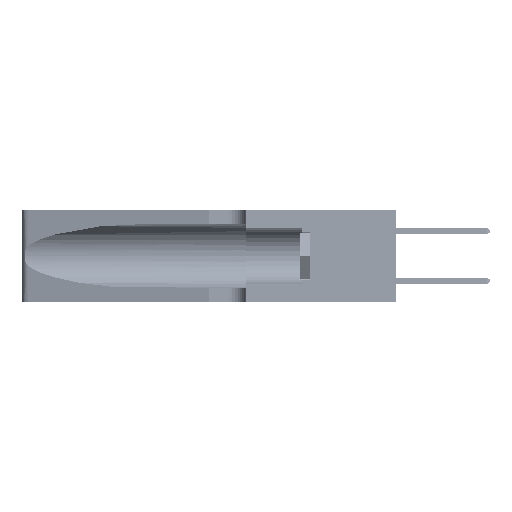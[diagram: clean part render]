
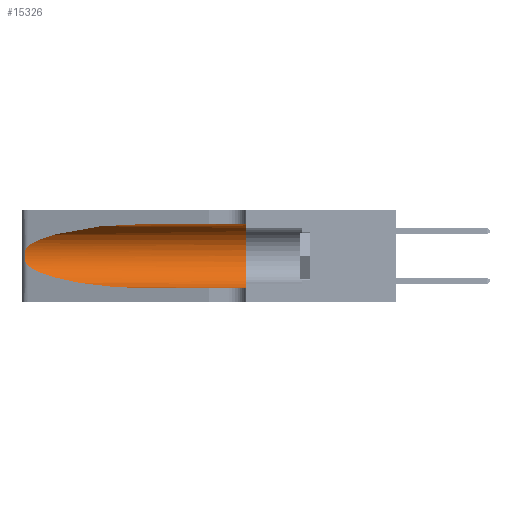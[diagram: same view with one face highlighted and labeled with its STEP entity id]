
A CAD part, left-side view. The second image highlights one B-rep face of the part: STEP entity #15326.
In plain terms, the highlighted cylindrical face has radius 3.308 mm (diameter 6.617 mm), a partial arc.
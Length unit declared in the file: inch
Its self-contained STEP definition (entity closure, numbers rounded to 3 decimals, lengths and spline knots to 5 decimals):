
#369 = CARTESIAN_POINT ( 'NONE',  ( 0.18966, 0.96281, 0.05475 ) ) ;
#538 = AXIS2_PLACEMENT_3D ( 'NONE', #7253, #50254, #26796 ) ;
#1920 = CARTESIAN_POINT ( 'NONE',  ( 0.1305, 0.72297, 0.05475 ) ) ;
#3194 = ORIENTED_EDGE ( 'NONE', *, *, #28924, .T. ) ;
#3664 = ORIENTED_EDGE ( 'NONE', *, *, #30258, .T. ) ;
#4089 = CARTESIAN_POINT ( 'NONE',  ( 0.26075, 1.23896, 0.19203 ) ) ;
#4141 = CARTESIAN_POINT ( 'NONE',  ( 0.25487, 1.22718, 0.14631 ) ) ;
#4428 = CARTESIAN_POINT ( 'NONE',  ( 0.25487, 1.22718, 0.22369 ) ) ;
#5025 = FACE_OUTER_BOUND ( 'NONE', #24819, .T. ) ;
#7253 = CARTESIAN_POINT ( 'NONE',  ( 0.1305, 0.35, 0.185 ) ) ;
#8029 = CARTESIAN_POINT ( 'NONE',  ( 0.25639, 1.23184, 0.21858 ) ) ;
#8126 = EDGE_CURVE ( 'NONE', #20745, #47649, #30087, .T. ) ;
#8811 = VERTEX_POINT ( 'NONE', #24138 ) ;
#9711 = DIRECTION ( 'NONE',  ( 0., -1., 0. ) ) ;
#10299 =( BOUNDED_CURVE ( )  B_SPLINE_CURVE ( 3, ( #44788, #48866, #36911, #29019 ),
 .UNSPECIFIED., .F., .T. ) 
 B_SPLINE_CURVE_WITH_KNOTS ( ( 4, 4 ),
 ( 1.5708, 2.84003 ),
 .UNSPECIFIED. ) 
 CURVE ( )  GEOMETRIC_REPRESENTATION_ITEM ( )  RATIONAL_B_SPLINE_CURVE ( ( 1., 0.87, 0.87, 1. ) ) 
 REPRESENTATION_ITEM ( '' )  );
#10627 = ORIENTED_EDGE ( 'NONE', *, *, #34378, .T. ) ;
#11359 = CIRCLE ( 'NONE', #538, 0.13025 ) ;
#11655 = CARTESIAN_POINT ( 'NONE',  ( 0.25789, 1.23486, 0.15765 ) ) ;
#11983 = VECTOR ( 'NONE', #9711, 39.37008 ) ;
#11985 = CARTESIAN_POINT ( 'NONE',  ( 0.25787, 1.23484, 0.2124 ) ) ;
#13602 = CYLINDRICAL_SURFACE ( 'NONE', #38420, 0.13025 ) ;
#15326 = ADVANCED_FACE ( 'NONE', ( #5025 ), #13602, .F. ) ;
#15617 = ORIENTED_EDGE ( 'NONE', *, *, #8126, .T. ) ;
#15785 = CARTESIAN_POINT ( 'NONE',  ( 0.26017, 1.23833, 0.17102 ) ) ;
#16115 = CARTESIAN_POINT ( 'NONE',  ( 0.25639, 1.23186, 0.15144 ) ) ;
#19671 = EDGE_CURVE ( 'NONE', #36906, #35275, #37132, .T. ) ;
#19709 = CARTESIAN_POINT ( 'NONE',  ( 0.25854, 1.2359, 0.20912 ) ) ;
#20040 = CARTESIAN_POINT ( 'NONE',  ( 0.26075, 1.23896, 0.178 ) ) ;
#20745 = VERTEX_POINT ( 'NONE', #4141 ) ;
#21710 = CARTESIAN_POINT ( 'NONE',  ( 0.1305, 1.61858, 0.31525 ) ) ;
#24138 = CARTESIAN_POINT ( 'NONE',  ( 0.25487, 1.22718, 0.22369 ) ) ;
#24819 = EDGE_LOOP ( 'NONE', ( #10627, #3664, #15617, #3194, #42760, #45668 ) ) ;
#25859 = CARTESIAN_POINT ( 'NONE',  ( 0.1305, 0.35, 0.05475 ) ) ;
#25973 = DIRECTION ( 'NONE',  ( 0., -1., 0. ) ) ;
#26796 = DIRECTION ( 'NONE',  ( 0., 0., 1. ) ) ;
#28157 = CARTESIAN_POINT ( 'NONE',  ( 0.1305, 0.72297, 0.31525 ) ) ;
#28924 = EDGE_CURVE ( 'NONE', #47649, #46301, #38168, .T. ) ;
#29019 = CARTESIAN_POINT ( 'NONE',  ( 0.25487, 1.22718, 0.22369 ) ) ;
#30087 =( BOUNDED_CURVE ( )  B_SPLINE_CURVE ( 3, ( #43939, #47710, #369, #35712 ),
 .UNSPECIFIED., .F., .T. ) 
 B_SPLINE_CURVE_WITH_KNOTS ( ( 4, 4 ),
 ( 3.44316, 4.71239 ),
 .UNSPECIFIED. ) 
 CURVE ( )  GEOMETRIC_REPRESENTATION_ITEM ( )  RATIONAL_B_SPLINE_CURVE ( ( 1., 0.87, 0.87, 1. ) ) 
 REPRESENTATION_ITEM ( '' )  );
#30258 = EDGE_CURVE ( 'NONE', #8811, #20745, #33272, .T. ) ;
#33272 = B_SPLINE_CURVE_WITH_KNOTS ( 'NONE', 3,
 ( #4428, #39266, #8029, #11985, #19709, #35308, #4089, #20040, #15785, #35802, #11655, #16115, #43198, #35477 ),
 .UNSPECIFIED., .F., .F.,
 ( 4, 2, 2, 2, 2, 2, 4 ),
 ( 0., 0.00027, 0.00053, 0.00107, 0.0016, 0.00187, 0.00214 ),
 .UNSPECIFIED. ) ;
#34378 = EDGE_CURVE ( 'NONE', #36906, #8811, #10299, .T. ) ;
#34650 = DIRECTION ( 'NONE',  ( 0., -1., 0. ) ) ;
#35275 = VERTEX_POINT ( 'NONE', #37871 ) ;
#35308 = CARTESIAN_POINT ( 'NONE',  ( 0.26018, 1.23835, 0.19895 ) ) ;
#35477 = CARTESIAN_POINT ( 'NONE',  ( 0.25487, 1.22718, 0.14631 ) ) ;
#35712 = CARTESIAN_POINT ( 'NONE',  ( 0.1305, 0.72297, 0.05475 ) ) ;
#35802 = CARTESIAN_POINT ( 'NONE',  ( 0.25856, 1.23593, 0.16098 ) ) ;
#36725 = EDGE_CURVE ( 'NONE', #35275, #46301, #11359, .T. ) ;
#36906 = VERTEX_POINT ( 'NONE', #28157 ) ;
#36911 = CARTESIAN_POINT ( 'NONE',  ( 0.2373, 1.15595, 0.28018 ) ) ;
#36993 = CARTESIAN_POINT ( 'NONE',  ( 0.1305, 1.61858, 0.185 ) ) ;
#37132 = LINE ( 'NONE', #21710, #11983 ) ;
#37680 = DIRECTION ( 'NONE',  ( 0., 0., -1. ) ) ;
#37871 = CARTESIAN_POINT ( 'NONE',  ( 0.1305, 0.35, 0.31525 ) ) ;
#38168 = LINE ( 'NONE', #50068, #49770 ) ;
#38420 = AXIS2_PLACEMENT_3D ( 'NONE', #36993, #25973, #37680 ) ;
#39266 = CARTESIAN_POINT ( 'NONE',  ( 0.25555, 1.22994, 0.2215 ) ) ;
#42760 = ORIENTED_EDGE ( 'NONE', *, *, #36725, .F. ) ;
#43198 = CARTESIAN_POINT ( 'NONE',  ( 0.25555, 1.22993, 0.14849 ) ) ;
#43939 = CARTESIAN_POINT ( 'NONE',  ( 0.25487, 1.22718, 0.14631 ) ) ;
#44788 = CARTESIAN_POINT ( 'NONE',  ( 0.1305, 0.72297, 0.31525 ) ) ;
#45668 = ORIENTED_EDGE ( 'NONE', *, *, #19671, .F. ) ;
#46301 = VERTEX_POINT ( 'NONE', #25859 ) ;
#47649 = VERTEX_POINT ( 'NONE', #1920 ) ;
#47710 = CARTESIAN_POINT ( 'NONE',  ( 0.2373, 1.15595, 0.08982 ) ) ;
#48866 = CARTESIAN_POINT ( 'NONE',  ( 0.18966, 0.96281, 0.31525 ) ) ;
#49770 = VECTOR ( 'NONE', #34650, 39.37008 ) ;
#50068 = CARTESIAN_POINT ( 'NONE',  ( 0.1305, 1.61858, 0.05475 ) ) ;
#50254 = DIRECTION ( 'NONE',  ( 0., 1., 0. ) ) ;
